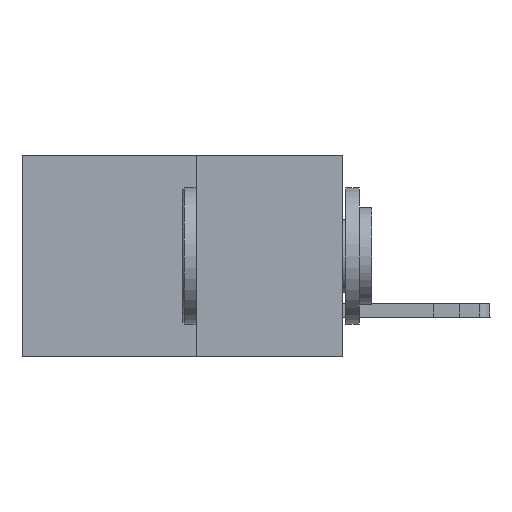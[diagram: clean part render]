
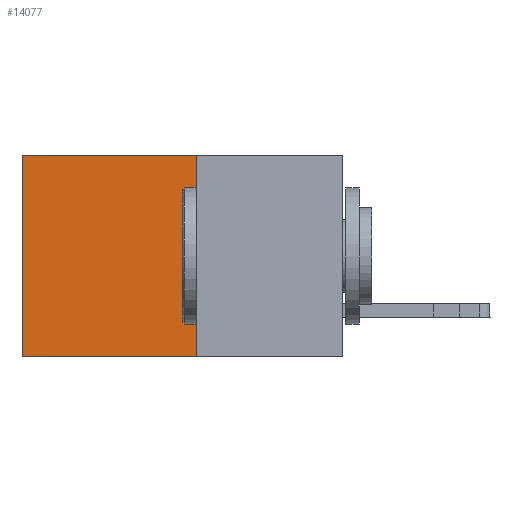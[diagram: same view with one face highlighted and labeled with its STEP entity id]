
A CAD part, left-side view. The second image highlights one B-rep face of the part: STEP entity #14077.
In plain terms, the highlighted planar face has unit normal (-1, 0, 0).
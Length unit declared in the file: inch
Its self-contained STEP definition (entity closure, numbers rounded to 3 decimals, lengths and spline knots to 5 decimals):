
#1026 = CARTESIAN_POINT ( 'NONE',  ( 0.277, 0.27, -0.37 ) ) ;
#1124 = VECTOR ( 'NONE', #9652, 39.37008 ) ;
#1844 = VECTOR ( 'NONE', #28700, 39.37008 ) ;
#2129 = ORIENTED_EDGE ( 'NONE', *, *, #14732, .F. ) ;
#2176 = DIRECTION ( 'NONE',  ( 0., 1., 0. ) ) ;
#3723 = VECTOR ( 'NONE', #2176, 39.37008 ) ;
#5687 = VERTEX_POINT ( 'NONE', #29760 ) ;
#7059 = CARTESIAN_POINT ( 'NONE',  ( 0.277, 0.27, -0.37 ) ) ;
#8387 = CARTESIAN_POINT ( 'NONE',  ( 0.277, 0.27, 0. ) ) ;
#8438 = DIRECTION ( 'NONE',  ( 1., 0., 0. ) ) ;
#9450 = LINE ( 'NONE', #17057, #3723 ) ;
#9652 = DIRECTION ( 'NONE',  ( 0., 0., -1. ) ) ;
#10343 = ORIENTED_EDGE ( 'NONE', *, *, #24157, .F. ) ;
#11027 = DIRECTION ( 'NONE',  ( 0., 0., -1. ) ) ;
#13202 = VECTOR ( 'NONE', #14635, 39.37008 ) ;
#13674 = LINE ( 'NONE', #23538, #1844 ) ;
#14077 = ADVANCED_FACE ( 'NONE', ( #15576 ), #30582, .F. ) ;
#14635 = DIRECTION ( 'NONE',  ( 0., 0., -1. ) ) ;
#14732 = EDGE_CURVE ( 'NONE', #19974, #20035, #16932, .T. ) ;
#15576 = FACE_OUTER_BOUND ( 'NONE', #25045, .T. ) ;
#16932 = LINE ( 'NONE', #7059, #1124 ) ;
#17057 = CARTESIAN_POINT ( 'NONE',  ( 0.277, 0.27, -0.37 ) ) ;
#18732 = CARTESIAN_POINT ( 'NONE',  ( 0.277, 0.27, -0.37 ) ) ;
#19974 = VERTEX_POINT ( 'NONE', #8387 ) ;
#20035 = VERTEX_POINT ( 'NONE', #18732 ) ;
#20096 = CARTESIAN_POINT ( 'NONE',  ( 0.277, 0.59, 0. ) ) ;
#21913 = LINE ( 'NONE', #29173, #13202 ) ;
#23538 = CARTESIAN_POINT ( 'NONE',  ( 0.277, 0.27, 0. ) ) ;
#24157 = EDGE_CURVE ( 'NONE', #20035, #5687, #9450, .T. ) ;
#25045 = EDGE_LOOP ( 'NONE', ( #27032, #10343, #2129, #27812 ) ) ;
#27032 = ORIENTED_EDGE ( 'NONE', *, *, #28670, .T. ) ;
#27794 = VERTEX_POINT ( 'NONE', #20096 ) ;
#27812 = ORIENTED_EDGE ( 'NONE', *, *, #28542, .T. ) ;
#28542 = EDGE_CURVE ( 'NONE', #19974, #27794, #13674, .T. ) ;
#28670 = EDGE_CURVE ( 'NONE', #27794, #5687, #21913, .T. ) ;
#28700 = DIRECTION ( 'NONE',  ( 0., 1., 0. ) ) ;
#29173 = CARTESIAN_POINT ( 'NONE',  ( 0.277, 0.59, -0.37 ) ) ;
#29760 = CARTESIAN_POINT ( 'NONE',  ( 0.277, 0.59, -0.37 ) ) ;
#29983 = AXIS2_PLACEMENT_3D ( 'NONE', #1026, #8438, #11027 ) ;
#30582 = PLANE ( 'NONE',  #29983 ) ;
